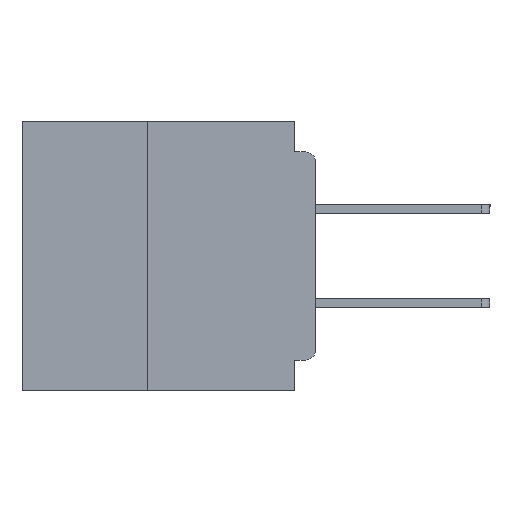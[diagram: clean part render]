
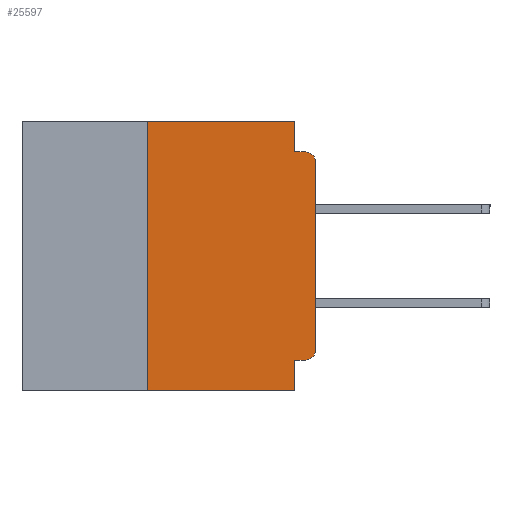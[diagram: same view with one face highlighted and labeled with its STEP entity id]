
A CAD part, left-side view. The second image highlights one B-rep face of the part: STEP entity #25597.
In plain terms, the highlighted planar face has unit normal (-1, 0, 0).
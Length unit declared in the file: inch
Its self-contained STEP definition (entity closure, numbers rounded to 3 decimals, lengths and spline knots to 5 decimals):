
#88 = VECTOR ( 'NONE', #28449, 39.37008 ) ;
#204 = VERTEX_POINT ( 'NONE', #30118 ) ;
#1085 = CIRCLE ( 'NONE', #9787, 0.015 ) ;
#1163 = VECTOR ( 'NONE', #30665, 39.37008 ) ;
#1208 = ORIENTED_EDGE ( 'NONE', *, *, #16320, .T. ) ;
#1224 = CARTESIAN_POINT ( 'NONE',  ( 0., 0.031, -0.4 ) ) ;
#1785 = CARTESIAN_POINT ( 'NONE',  ( 0., 0.015, -0.045 ) ) ;
#2225 = CARTESIAN_POINT ( 'NONE',  ( 0., 0.25, -0.4 ) ) ;
#2572 = FACE_OUTER_BOUND ( 'NONE', #22290, .T. ) ;
#2682 = LINE ( 'NONE', #24752, #9646 ) ;
#2971 = LINE ( 'NONE', #10722, #18714 ) ;
#3061 = EDGE_CURVE ( 'NONE', #21931, #10658, #5541, .T. ) ;
#3173 = VERTEX_POINT ( 'NONE', #2225 ) ;
#3287 = LINE ( 'NONE', #8794, #26964 ) ;
#3554 = ORIENTED_EDGE ( 'NONE', *, *, #5747, .T. ) ;
#4634 = VERTEX_POINT ( 'NONE', #20025 ) ;
#4720 = CARTESIAN_POINT ( 'NONE',  ( 0., 0.437, 0. ) ) ;
#4826 = EDGE_CURVE ( 'NONE', #3173, #204, #9112, .T. ) ;
#5497 = PLANE ( 'NONE',  #30101 ) ;
#5541 = LINE ( 'NONE', #9848, #36944 ) ;
#5747 = EDGE_CURVE ( 'NONE', #23917, #10658, #1085, .T. ) ;
#6534 = EDGE_CURVE ( 'NONE', #24279, #23917, #14168, .T. ) ;
#6828 = EDGE_CURVE ( 'NONE', #16116, #21931, #2971, .T. ) ;
#7775 = LINE ( 'NONE', #1224, #22556 ) ;
#8198 = ORIENTED_EDGE ( 'NONE', *, *, #3061, .F. ) ;
#8498 = CARTESIAN_POINT ( 'NONE',  ( 0., 0.015, -0.34 ) ) ;
#8794 = CARTESIAN_POINT ( 'NONE',  ( 0., 0.25, -0.4 ) ) ;
#9112 = LINE ( 'NONE', #30995, #1163 ) ;
#9646 = VECTOR ( 'NONE', #21917, 39.37008 ) ;
#9787 = AXIS2_PLACEMENT_3D ( 'NONE', #11978, #11864, #11775 ) ;
#9848 = CARTESIAN_POINT ( 'NONE',  ( 0., 0., -0.045 ) ) ;
#10096 = CIRCLE ( 'NONE', #25408, 0.015 ) ;
#10158 = ORIENTED_EDGE ( 'NONE', *, *, #6828, .F. ) ;
#10515 = CARTESIAN_POINT ( 'NONE',  ( 0., 0.25, 0. ) ) ;
#10658 = VERTEX_POINT ( 'NONE', #1785 ) ;
#10722 = CARTESIAN_POINT ( 'NONE',  ( 0., 0.031, 0. ) ) ;
#10768 = DIRECTION ( 'NONE',  ( 0., 0., -1. ) ) ;
#10847 = DIRECTION ( 'NONE',  ( 0., -1., 0. ) ) ;
#10860 = CARTESIAN_POINT ( 'NONE',  ( 0., 0.031, -0.045 ) ) ;
#10896 = ORIENTED_EDGE ( 'NONE', *, *, #4826, .T. ) ;
#10904 = EDGE_CURVE ( 'NONE', #3173, #11334, #3287, .T. ) ;
#11334 = VERTEX_POINT ( 'NONE', #10515 ) ;
#11494 = DIRECTION ( 'NONE',  ( 1., 0., 0. ) ) ;
#11520 = DIRECTION ( 'NONE',  ( 0., 0., -1. ) ) ;
#11775 = DIRECTION ( 'NONE',  ( 0., 0., -1. ) ) ;
#11864 = DIRECTION ( 'NONE',  ( -1., 0., 0. ) ) ;
#11978 = CARTESIAN_POINT ( 'NONE',  ( 0., 0.015, -0.06 ) ) ;
#14168 = LINE ( 'NONE', #24362, #21092 ) ;
#15029 = ORIENTED_EDGE ( 'NONE', *, *, #10904, .F. ) ;
#16116 = VERTEX_POINT ( 'NONE', #28228 ) ;
#16234 = CARTESIAN_POINT ( 'NONE',  ( 0., 0., -0.34 ) ) ;
#16320 = EDGE_CURVE ( 'NONE', #17310, #24279, #10096, .T. ) ;
#17310 = VERTEX_POINT ( 'NONE', #18906 ) ;
#18714 = VECTOR ( 'NONE', #10768, 39.37008 ) ;
#18906 = CARTESIAN_POINT ( 'NONE',  ( 0., 0.015, -0.355 ) ) ;
#20025 = CARTESIAN_POINT ( 'NONE',  ( 0., 0.031, -0.355 ) ) ;
#20204 = ORIENTED_EDGE ( 'NONE', *, *, #24710, .F. ) ;
#20411 = CARTESIAN_POINT ( 'NONE',  ( 0., 0., -0.06 ) ) ;
#21092 = VECTOR ( 'NONE', #24103, 39.37008 ) ;
#21917 = DIRECTION ( 'NONE',  ( 0., 1., 0. ) ) ;
#21931 = VERTEX_POINT ( 'NONE', #10860 ) ;
#22215 = ORIENTED_EDGE ( 'NONE', *, *, #6534, .T. ) ;
#22290 = EDGE_LOOP ( 'NONE', ( #22215, #3554, #8198, #10158, #25688, #15029, #10896, #20204, #27134, #1208 ) ) ;
#22556 = VECTOR ( 'NONE', #24977, 39.37008 ) ;
#23917 = VERTEX_POINT ( 'NONE', #20411 ) ;
#24103 = DIRECTION ( 'NONE',  ( 0., 0., 1. ) ) ;
#24216 = EDGE_CURVE ( 'NONE', #17310, #4634, #2682, .T. ) ;
#24279 = VERTEX_POINT ( 'NONE', #16234 ) ;
#24362 = CARTESIAN_POINT ( 'NONE',  ( 0., 0., 0. ) ) ;
#24710 = EDGE_CURVE ( 'NONE', #4634, #204, #7775, .T. ) ;
#24752 = CARTESIAN_POINT ( 'NONE',  ( 0., 0., -0.355 ) ) ;
#24977 = DIRECTION ( 'NONE',  ( 0., 0., -1. ) ) ;
#25408 = AXIS2_PLACEMENT_3D ( 'NONE', #8498, #29247, #11520 ) ;
#25597 = ADVANCED_FACE ( 'NONE', ( #2572 ), #5497, .F. ) ;
#25688 = ORIENTED_EDGE ( 'NONE', *, *, #35347, .F. ) ;
#26964 = VECTOR ( 'NONE', #29532, 39.37008 ) ;
#27134 = ORIENTED_EDGE ( 'NONE', *, *, #24216, .F. ) ;
#28228 = CARTESIAN_POINT ( 'NONE',  ( 0., 0.031, 0. ) ) ;
#28449 = DIRECTION ( 'NONE',  ( 0., -1., 0. ) ) ;
#29247 = DIRECTION ( 'NONE',  ( -1., 0., 0. ) ) ;
#29532 = DIRECTION ( 'NONE',  ( 0., 0., 1. ) ) ;
#30101 = AXIS2_PLACEMENT_3D ( 'NONE', #37855, #11494, #32180 ) ;
#30118 = CARTESIAN_POINT ( 'NONE',  ( 0., 0.031, -0.4 ) ) ;
#30665 = DIRECTION ( 'NONE',  ( 0., -1., 0. ) ) ;
#30995 = CARTESIAN_POINT ( 'NONE',  ( 0., 0.437, -0.4 ) ) ;
#31704 = LINE ( 'NONE', #4720, #88 ) ;
#32180 = DIRECTION ( 'NONE',  ( 0., 0., -1. ) ) ;
#35347 = EDGE_CURVE ( 'NONE', #11334, #16116, #31704, .T. ) ;
#36944 = VECTOR ( 'NONE', #10847, 39.37008 ) ;
#37855 = CARTESIAN_POINT ( 'NONE',  ( 0., 0.437, 0. ) ) ;
